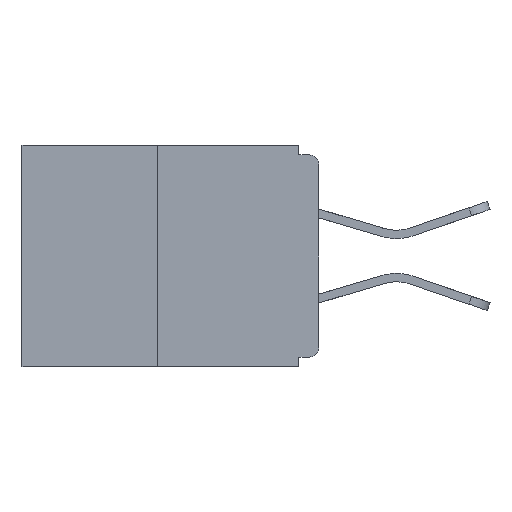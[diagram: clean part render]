
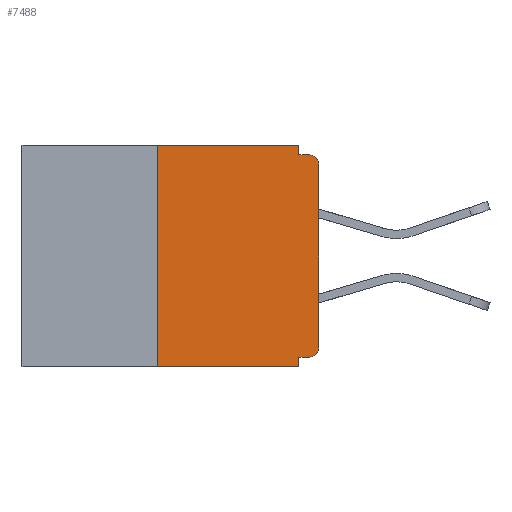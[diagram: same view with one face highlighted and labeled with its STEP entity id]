
A CAD part, left-side view. The second image highlights one B-rep face of the part: STEP entity #7488.
In plain terms, the highlighted planar face has unit normal (-1, 0, 0).
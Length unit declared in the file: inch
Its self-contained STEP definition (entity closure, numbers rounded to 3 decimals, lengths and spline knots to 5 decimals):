
#431 = CARTESIAN_POINT ( 'NONE',  ( 0., 0.031, 0. ) ) ;
#747 = ORIENTED_EDGE ( 'NONE', *, *, #19437, .F. ) ;
#1081 = CARTESIAN_POINT ( 'NONE',  ( 0., 0.25, 0. ) ) ;
#1117 = VECTOR ( 'NONE', #14897, 39.37008 ) ;
#1174 = VECTOR ( 'NONE', #6947, 39.37008 ) ;
#1379 = EDGE_LOOP ( 'NONE', ( #5286, #21294, #7068, #10709, #4329, #8328, #12468, #2477, #9019, #747 ) ) ;
#1415 = CARTESIAN_POINT ( 'NONE',  ( 0., 0., -0.03 ) ) ;
#1803 = PLANE ( 'NONE',  #20314 ) ;
#2124 = VECTOR ( 'NONE', #11060, 39.37008 ) ;
#2388 = EDGE_CURVE ( 'NONE', #6198, #12955, #15654, .T. ) ;
#2477 = ORIENTED_EDGE ( 'NONE', *, *, #3256, .T. ) ;
#2778 = CARTESIAN_POINT ( 'NONE',  ( 0., 0.25, 0. ) ) ;
#2847 = DIRECTION ( 'NONE',  ( 0., 0., -1. ) ) ;
#2852 = CIRCLE ( 'NONE', #13626, 0.015 ) ;
#2930 = VERTEX_POINT ( 'NONE', #6365 ) ;
#3256 = EDGE_CURVE ( 'NONE', #12955, #18039, #2852, .T. ) ;
#3347 = VERTEX_POINT ( 'NONE', #6127 ) ;
#3944 = CARTESIAN_POINT ( 'NONE',  ( 0., 0.031, -0.343 ) ) ;
#4299 = DIRECTION ( 'NONE',  ( 0., 0., 1. ) ) ;
#4329 = ORIENTED_EDGE ( 'NONE', *, *, #7794, .F. ) ;
#4348 = CIRCLE ( 'NONE', #13758, 0.015 ) ;
#4704 = DIRECTION ( 'NONE',  ( 0., -1., 0. ) ) ;
#4814 = LINE ( 'NONE', #12961, #19764 ) ;
#5286 = ORIENTED_EDGE ( 'NONE', *, *, #11580, .F. ) ;
#6127 = CARTESIAN_POINT ( 'NONE',  ( 0., 0.015, -0.328 ) ) ;
#6198 = VERTEX_POINT ( 'NONE', #15205 ) ;
#6269 = VERTEX_POINT ( 'NONE', #11598 ) ;
#6365 = CARTESIAN_POINT ( 'NONE',  ( 0., 0.031, -0.328 ) ) ;
#6761 = VERTEX_POINT ( 'NONE', #3944 ) ;
#6850 = CARTESIAN_POINT ( 'NONE',  ( 0., 0.015, -0.015 ) ) ;
#6947 = DIRECTION ( 'NONE',  ( 0., -1., 0. ) ) ;
#7068 = ORIENTED_EDGE ( 'NONE', *, *, #7394, .T. ) ;
#7394 = EDGE_CURVE ( 'NONE', #6269, #6761, #16073, .T. ) ;
#7488 = ADVANCED_FACE ( 'NONE', ( #16399 ), #1803, .F. ) ;
#7627 = VERTEX_POINT ( 'NONE', #15318 ) ;
#7778 = CARTESIAN_POINT ( 'NONE',  ( 0., 0., -0.328 ) ) ;
#7790 = LINE ( 'NONE', #2778, #15160 ) ;
#7794 = EDGE_CURVE ( 'NONE', #3347, #2930, #11251, .T. ) ;
#8133 = DIRECTION ( 'NONE',  ( 1., 0., 0. ) ) ;
#8328 = ORIENTED_EDGE ( 'NONE', *, *, #8725, .T. ) ;
#8457 = CARTESIAN_POINT ( 'NONE',  ( 0., 0.46, 0. ) ) ;
#8578 = VECTOR ( 'NONE', #11202, 39.37008 ) ;
#8725 = EDGE_CURVE ( 'NONE', #3347, #6198, #4348, .T. ) ;
#9019 = ORIENTED_EDGE ( 'NONE', *, *, #17216, .F. ) ;
#9579 = CARTESIAN_POINT ( 'NONE',  ( 0., 0.031, -0.343 ) ) ;
#9770 = EDGE_CURVE ( 'NONE', #2930, #6761, #19397, .T. ) ;
#9992 = LINE ( 'NONE', #13164, #1117 ) ;
#10709 = ORIENTED_EDGE ( 'NONE', *, *, #9770, .F. ) ;
#11060 = DIRECTION ( 'NONE',  ( 0., 0., 1. ) ) ;
#11202 = DIRECTION ( 'NONE',  ( 0., 0., -1. ) ) ;
#11251 = LINE ( 'NONE', #7778, #16148 ) ;
#11253 = CARTESIAN_POINT ( 'NONE',  ( 0., 0.031, 0. ) ) ;
#11580 = EDGE_CURVE ( 'NONE', #16080, #12048, #9992, .T. ) ;
#11598 = CARTESIAN_POINT ( 'NONE',  ( 0., 0.25, -0.343 ) ) ;
#12048 = VERTEX_POINT ( 'NONE', #431 ) ;
#12468 = ORIENTED_EDGE ( 'NONE', *, *, #2388, .T. ) ;
#12955 = VERTEX_POINT ( 'NONE', #1415 ) ;
#12961 = CARTESIAN_POINT ( 'NONE',  ( 0., 0., -0.015 ) ) ;
#13090 = CARTESIAN_POINT ( 'NONE',  ( 0., 0.015, -0.03 ) ) ;
#13164 = CARTESIAN_POINT ( 'NONE',  ( 0., 0.46, 0. ) ) ;
#13626 = AXIS2_PLACEMENT_3D ( 'NONE', #13090, #17662, #2847 ) ;
#13758 = AXIS2_PLACEMENT_3D ( 'NONE', #20447, #15736, #15425 ) ;
#14447 = CARTESIAN_POINT ( 'NONE',  ( 0., 0.46, -0.343 ) ) ;
#14859 = DIRECTION ( 'NONE',  ( 0., 0., -1. ) ) ;
#14897 = DIRECTION ( 'NONE',  ( 0., -1., 0. ) ) ;
#15160 = VECTOR ( 'NONE', #4299, 39.37008 ) ;
#15205 = CARTESIAN_POINT ( 'NONE',  ( 0., 0., -0.313 ) ) ;
#15318 = CARTESIAN_POINT ( 'NONE',  ( 0., 0.031, -0.015 ) ) ;
#15425 = DIRECTION ( 'NONE',  ( 0., 0., -1. ) ) ;
#15654 = LINE ( 'NONE', #17492, #2124 ) ;
#15736 = DIRECTION ( 'NONE',  ( -1., 0., 0. ) ) ;
#16073 = LINE ( 'NONE', #14447, #1174 ) ;
#16080 = VERTEX_POINT ( 'NONE', #1081 ) ;
#16148 = VECTOR ( 'NONE', #21075, 39.37008 ) ;
#16274 = EDGE_CURVE ( 'NONE', #6269, #16080, #7790, .T. ) ;
#16374 = LINE ( 'NONE', #11253, #19421 ) ;
#16399 = FACE_OUTER_BOUND ( 'NONE', #1379, .T. ) ;
#16630 = DIRECTION ( 'NONE',  ( 0., 0., -1. ) ) ;
#17216 = EDGE_CURVE ( 'NONE', #7627, #18039, #4814, .T. ) ;
#17492 = CARTESIAN_POINT ( 'NONE',  ( 0., 0., 0. ) ) ;
#17662 = DIRECTION ( 'NONE',  ( -1., 0., 0. ) ) ;
#18039 = VERTEX_POINT ( 'NONE', #6850 ) ;
#19397 = LINE ( 'NONE', #9579, #8578 ) ;
#19421 = VECTOR ( 'NONE', #14859, 39.37008 ) ;
#19437 = EDGE_CURVE ( 'NONE', #12048, #7627, #16374, .T. ) ;
#19764 = VECTOR ( 'NONE', #4704, 39.37008 ) ;
#20314 = AXIS2_PLACEMENT_3D ( 'NONE', #8457, #8133, #16630 ) ;
#20447 = CARTESIAN_POINT ( 'NONE',  ( 0., 0.015, -0.313 ) ) ;
#21075 = DIRECTION ( 'NONE',  ( 0., 1., 0. ) ) ;
#21294 = ORIENTED_EDGE ( 'NONE', *, *, #16274, .F. ) ;
